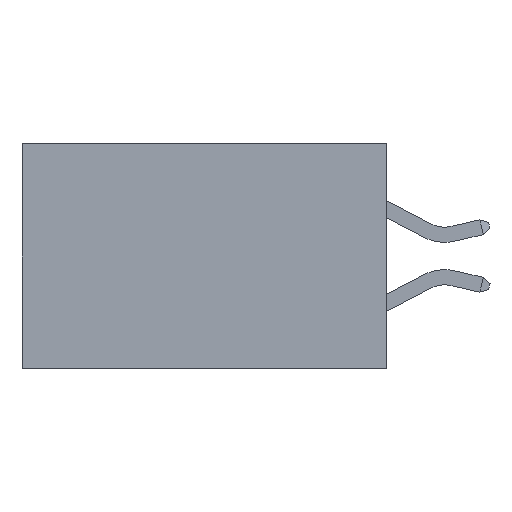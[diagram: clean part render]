
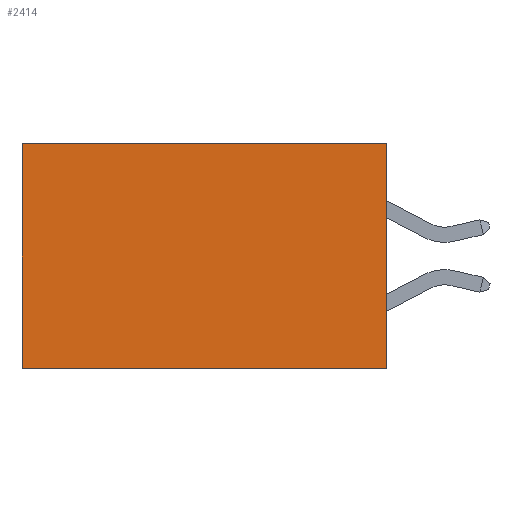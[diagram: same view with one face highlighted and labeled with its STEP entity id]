
A CAD part, left-side view. The second image highlights one B-rep face of the part: STEP entity #2414.
In plain terms, the highlighted planar face has unit normal (-1, 0, 0).
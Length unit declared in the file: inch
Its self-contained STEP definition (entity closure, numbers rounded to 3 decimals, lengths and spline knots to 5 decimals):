
#737 = ORIENTED_EDGE ( 'NONE', *, *, #9236, .T. ) ;
#1525 = LINE ( 'NONE', #18460, #5503 ) ;
#2414 = ADVANCED_FACE ( 'NONE', ( #18741 ), #17118, .F. ) ;
#2796 = VECTOR ( 'NONE', #4304, 39.37008 ) ;
#2816 = CARTESIAN_POINT ( 'NONE',  ( 0.2615, 0.6, -0.37 ) ) ;
#2876 = CARTESIAN_POINT ( 'NONE',  ( 0.2615, 0., 0. ) ) ;
#4081 = VECTOR ( 'NONE', #13619, 39.37008 ) ;
#4304 = DIRECTION ( 'NONE',  ( 0., 0., -1. ) ) ;
#5305 = EDGE_CURVE ( 'NONE', #13087, #9928, #1525, .T. ) ;
#5503 = VECTOR ( 'NONE', #18588, 39.37008 ) ;
#5761 = EDGE_LOOP ( 'NONE', ( #737, #7623, #8941, #11043 ) ) ;
#6322 = CARTESIAN_POINT ( 'NONE',  ( 0.2615, 0.6, 0. ) ) ;
#7623 = ORIENTED_EDGE ( 'NONE', *, *, #13109, .F. ) ;
#8941 = ORIENTED_EDGE ( 'NONE', *, *, #5305, .F. ) ;
#9236 = EDGE_CURVE ( 'NONE', #11261, #14497, #11136, .T. ) ;
#9928 = VERTEX_POINT ( 'NONE', #13905 ) ;
#10338 = CARTESIAN_POINT ( 'NONE',  ( 0.2615, 0., -0.37 ) ) ;
#10847 = AXIS2_PLACEMENT_3D ( 'NONE', #18356, #16904, #17278 ) ;
#11043 = ORIENTED_EDGE ( 'NONE', *, *, #13865, .T. ) ;
#11136 = LINE ( 'NONE', #2816, #2796 ) ;
#11261 = VERTEX_POINT ( 'NONE', #6322 ) ;
#12130 = CARTESIAN_POINT ( 'NONE',  ( 0.2615, 0., 0. ) ) ;
#13087 = VERTEX_POINT ( 'NONE', #2876 ) ;
#13109 = EDGE_CURVE ( 'NONE', #9928, #14497, #13645, .T. ) ;
#13619 = DIRECTION ( 'NONE',  ( 0., 1., 0. ) ) ;
#13645 = LINE ( 'NONE', #10338, #14564 ) ;
#13865 = EDGE_CURVE ( 'NONE', #13087, #11261, #15906, .T. ) ;
#13905 = CARTESIAN_POINT ( 'NONE',  ( 0.2615, 0., -0.37 ) ) ;
#14497 = VERTEX_POINT ( 'NONE', #14944 ) ;
#14564 = VECTOR ( 'NONE', #19172, 39.37008 ) ;
#14944 = CARTESIAN_POINT ( 'NONE',  ( 0.2615, 0.6, -0.37 ) ) ;
#15906 = LINE ( 'NONE', #12130, #4081 ) ;
#16904 = DIRECTION ( 'NONE',  ( 1., 0., 0. ) ) ;
#17118 = PLANE ( 'NONE',  #10847 ) ;
#17278 = DIRECTION ( 'NONE',  ( 0., 0., -1. ) ) ;
#18356 = CARTESIAN_POINT ( 'NONE',  ( 0.2615, 0., -0.37 ) ) ;
#18460 = CARTESIAN_POINT ( 'NONE',  ( 0.2615, 0., -0.37 ) ) ;
#18588 = DIRECTION ( 'NONE',  ( 0., 0., -1. ) ) ;
#18741 = FACE_OUTER_BOUND ( 'NONE', #5761, .T. ) ;
#19172 = DIRECTION ( 'NONE',  ( 0., 1., 0. ) ) ;
